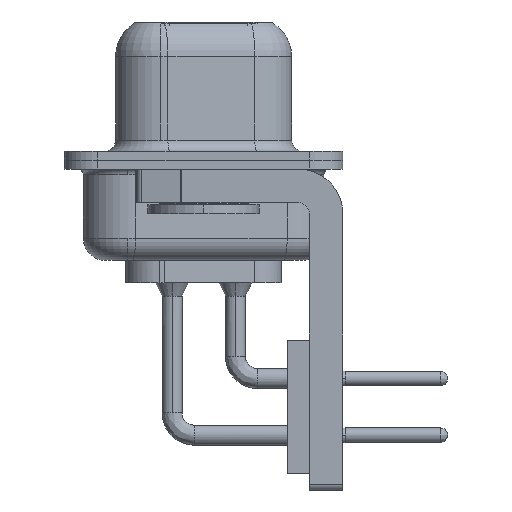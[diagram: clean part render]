
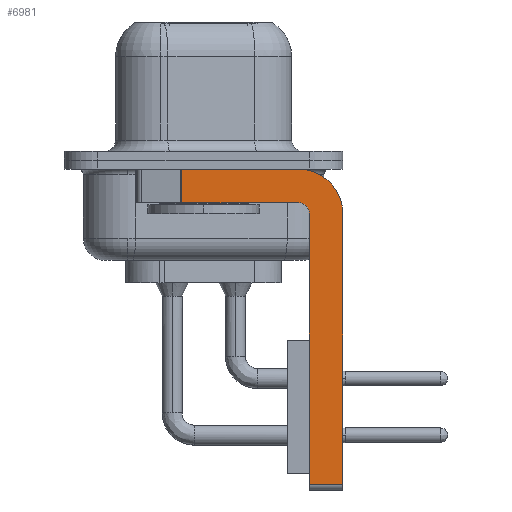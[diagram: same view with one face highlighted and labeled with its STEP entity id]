
A CAD part, left-side view. The second image highlights one B-rep face of the part: STEP entity #6981.
In plain terms, the highlighted planar face has unit normal (-1, 0, 0).
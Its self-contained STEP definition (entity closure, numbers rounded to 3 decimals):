
#145 = EDGE_CURVE ( 'NONE', #3989, #9236, #7102, .T. ) ;
#381 = CARTESIAN_POINT ( 'NONE',  ( -2.9, -4.25, -14.55 ) ) ;
#658 = EDGE_CURVE ( 'NONE', #9236, #5734, #11738, .T. ) ;
#952 = AXIS2_PLACEMENT_3D ( 'NONE', #6315, #17264, #7885 ) ;
#2223 = CARTESIAN_POINT ( 'NONE',  ( -2.9, -4.75, -2.4 ) ) ;
#2488 = LINE ( 'NONE', #381, #11345 ) ;
#2527 = CARTESIAN_POINT ( 'NONE',  ( -2.9, -6.25, -2.4 ) ) ;
#3633 = LINE ( 'NONE', #16091, #6363 ) ;
#3802 = CARTESIAN_POINT ( 'NONE',  ( -2.9, -4.75, -14.55 ) ) ;
#3989 = VERTEX_POINT ( 'NONE', #2223 ) ;
#4022 = DIRECTION ( 'NONE',  ( 0., 0., 1. ) ) ;
#4241 = VECTOR ( 'NONE', #18184, 1000. ) ;
#4768 = VERTEX_POINT ( 'NONE', #7482 ) ;
#4831 = CARTESIAN_POINT ( 'NONE',  ( -2.9, -4.25, -0.4 ) ) ;
#5444 = ORIENTED_EDGE ( 'NONE', *, *, #11432, .F. ) ;
#5734 = VERTEX_POINT ( 'NONE', #8178 ) ;
#6093 = DIRECTION ( 'NONE',  ( 0., 0., -1. ) ) ;
#6177 = EDGE_CURVE ( 'NONE', #9747, #4768, #7141, .T. ) ;
#6225 = VERTEX_POINT ( 'NONE', #18217 ) ;
#6315 = CARTESIAN_POINT ( 'NONE',  ( -2.9, -4.25, -2.4 ) ) ;
#6363 = VECTOR ( 'NONE', #6721, 1000. ) ;
#6721 = DIRECTION ( 'NONE',  ( 0., 0., 1. ) ) ;
#6981 = ADVANCED_FACE ( 'NONE', ( #7355 ), #9175, .F. ) ;
#7040 = DIRECTION ( 'NONE',  ( 0., -1., 0. ) ) ;
#7083 = VECTOR ( 'NONE', #8838, 1000. ) ;
#7102 = CIRCLE ( 'NONE', #12358, 0.5 ) ;
#7141 = LINE ( 'NONE', #2527, #10844 ) ;
#7253 = CARTESIAN_POINT ( 'NONE',  ( -2.9, -4.25, -2.4 ) ) ;
#7355 = FACE_OUTER_BOUND ( 'NONE', #15465, .T. ) ;
#7482 = CARTESIAN_POINT ( 'NONE',  ( -2.9, -6.25, -14.55 ) ) ;
#7647 = VERTEX_POINT ( 'NONE', #4831 ) ;
#7885 = DIRECTION ( 'NONE',  ( 0., 0., -1. ) ) ;
#8178 = CARTESIAN_POINT ( 'NONE',  ( -2.9, 0.978, -1.9 ) ) ;
#8382 = ORIENTED_EDGE ( 'NONE', *, *, #6177, .F. ) ;
#8458 = EDGE_CURVE ( 'NONE', #17959, #3989, #3633, .T. ) ;
#8838 = DIRECTION ( 'NONE',  ( 0., 1., 0. ) ) ;
#8899 = LINE ( 'NONE', #19722, #4241 ) ;
#9175 = PLANE ( 'NONE',  #12752 ) ;
#9236 = VERTEX_POINT ( 'NONE', #16601 ) ;
#9318 = DIRECTION ( 'NONE',  ( -1., 0., 0. ) ) ;
#9747 = VERTEX_POINT ( 'NONE', #13043 ) ;
#10370 = DIRECTION ( 'NONE',  ( 0., 0., -1. ) ) ;
#10648 = ORIENTED_EDGE ( 'NONE', *, *, #8458, .F. ) ;
#10844 = VECTOR ( 'NONE', #10370, 1000. ) ;
#11345 = VECTOR ( 'NONE', #11406, 1000. ) ;
#11406 = DIRECTION ( 'NONE',  ( 0., -1., 0. ) ) ;
#11432 = EDGE_CURVE ( 'NONE', #6225, #7647, #11648, .T. ) ;
#11648 = LINE ( 'NONE', #16425, #19449 ) ;
#11738 = LINE ( 'NONE', #14670, #7083 ) ;
#12258 = ORIENTED_EDGE ( 'NONE', *, *, #18883, .T. ) ;
#12328 = EDGE_CURVE ( 'NONE', #7647, #9747, #15716, .T. ) ;
#12358 = AXIS2_PLACEMENT_3D ( 'NONE', #7253, #9318, #4022 ) ;
#12752 = AXIS2_PLACEMENT_3D ( 'NONE', #20107, #15487, #6093 ) ;
#12980 = ORIENTED_EDGE ( 'NONE', *, *, #145, .F. ) ;
#13043 = CARTESIAN_POINT ( 'NONE',  ( -2.9, -6.25, -2.4 ) ) ;
#14670 = CARTESIAN_POINT ( 'NONE',  ( -2.9, -4.25, -1.9 ) ) ;
#15465 = EDGE_LOOP ( 'NONE', ( #5444, #12258, #19302, #12980, #10648, #15531, #8382, #17066 ) ) ;
#15487 = DIRECTION ( 'NONE',  ( 1., 0., 0. ) ) ;
#15531 = ORIENTED_EDGE ( 'NONE', *, *, #19266, .T. ) ;
#15716 = CIRCLE ( 'NONE', #952, 2. ) ;
#16091 = CARTESIAN_POINT ( 'NONE',  ( -2.9, -4.75, -14.8 ) ) ;
#16425 = CARTESIAN_POINT ( 'NONE',  ( -2.9, 3., -0.4 ) ) ;
#16601 = CARTESIAN_POINT ( 'NONE',  ( -2.9, -4.25, -1.9 ) ) ;
#17066 = ORIENTED_EDGE ( 'NONE', *, *, #12328, .F. ) ;
#17264 = DIRECTION ( 'NONE',  ( 1., 0., 0. ) ) ;
#17959 = VERTEX_POINT ( 'NONE', #3802 ) ;
#18184 = DIRECTION ( 'NONE',  ( 0., 0., -1. ) ) ;
#18217 = CARTESIAN_POINT ( 'NONE',  ( -2.9, 0.978, -0.4 ) ) ;
#18883 = EDGE_CURVE ( 'NONE', #6225, #5734, #8899, .T. ) ;
#19266 = EDGE_CURVE ( 'NONE', #17959, #4768, #2488, .T. ) ;
#19302 = ORIENTED_EDGE ( 'NONE', *, *, #658, .F. ) ;
#19449 = VECTOR ( 'NONE', #7040, 1000. ) ;
#19722 = CARTESIAN_POINT ( 'NONE',  ( -2.9, 0.978, -1.9 ) ) ;
#20107 = CARTESIAN_POINT ( 'NONE',  ( -2.9, -4.25, -2.4 ) ) ;
